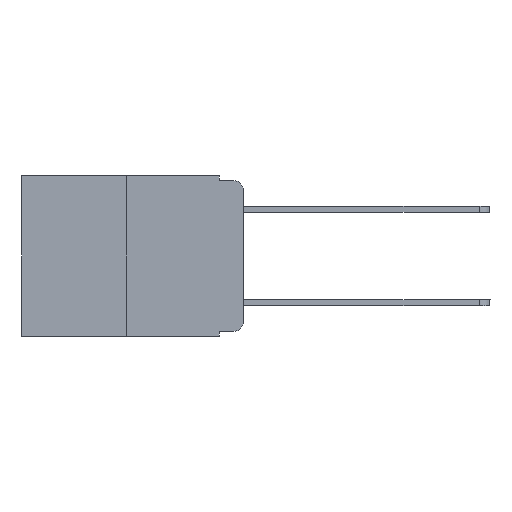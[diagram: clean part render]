
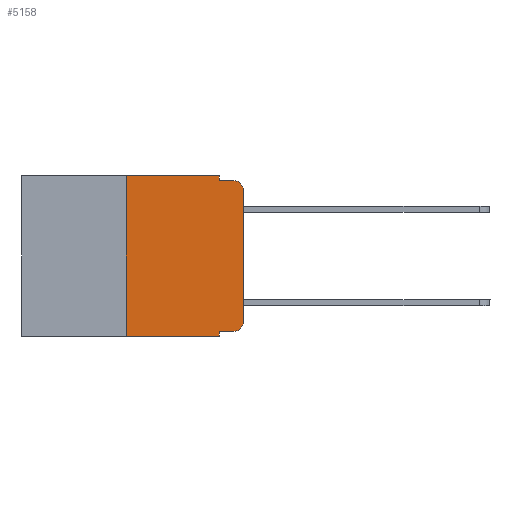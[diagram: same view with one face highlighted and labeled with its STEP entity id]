
A CAD part, left-side view. The second image highlights one B-rep face of the part: STEP entity #5158.
In plain terms, the highlighted planar face has unit normal (-1, 0, 0).
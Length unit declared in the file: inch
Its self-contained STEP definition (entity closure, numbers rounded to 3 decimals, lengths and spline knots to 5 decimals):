
#321 = EDGE_CURVE ( 'NONE', #15017, #14104, #5727, .T. ) ;
#492 = ORIENTED_EDGE ( 'NONE', *, *, #1290, .T. ) ;
#833 = ORIENTED_EDGE ( 'NONE', *, *, #7509, .F. ) ;
#1290 = EDGE_CURVE ( 'NONE', #7722, #4418, #1539, .T. ) ;
#1388 = CARTESIAN_POINT ( 'NONE',  ( 0., 0.051, -0.333 ) ) ;
#1406 = DIRECTION ( 'NONE',  ( -1., 0., 0. ) ) ;
#1539 = LINE ( 'NONE', #12666, #15130 ) ;
#1644 = VECTOR ( 'NONE', #11924, 39.37008 ) ;
#1881 = CARTESIAN_POINT ( 'NONE',  ( 0., 0., 0. ) ) ;
#1985 = FACE_OUTER_BOUND ( 'NONE', #8503, .T. ) ;
#3303 = EDGE_CURVE ( 'NONE', #15473, #14909, #5227, .T. ) ;
#3491 = CARTESIAN_POINT ( 'NONE',  ( 0., 0.02, -0.01 ) ) ;
#3507 = LINE ( 'NONE', #1388, #11747 ) ;
#3516 = AXIS2_PLACEMENT_3D ( 'NONE', #14765, #1406, #15905 ) ;
#4091 = DIRECTION ( 'NONE',  ( 0., -1., 0. ) ) ;
#4334 = CARTESIAN_POINT ( 'NONE',  ( 0., 0.051, 0. ) ) ;
#4418 = VERTEX_POINT ( 'NONE', #13692 ) ;
#4553 = DIRECTION ( 'NONE',  ( 0., -1., 0. ) ) ;
#4775 = CARTESIAN_POINT ( 'NONE',  ( 0., 0.02, -0.333 ) ) ;
#5158 = ADVANCED_FACE ( 'NONE', ( #1985 ), #9285, .F. ) ;
#5227 = LINE ( 'NONE', #11128, #7269 ) ;
#5446 = CARTESIAN_POINT ( 'NONE',  ( 0., 0.25, -0.343 ) ) ;
#5560 = ORIENTED_EDGE ( 'NONE', *, *, #16649, .F. ) ;
#5727 = CIRCLE ( 'NONE', #3516, 0.02 ) ;
#6538 = DIRECTION ( 'NONE',  ( 0., 0., 1. ) ) ;
#6646 = DIRECTION ( 'NONE',  ( 0., 0., -1. ) ) ;
#6820 = DIRECTION ( 'NONE',  ( 0., 0., -1. ) ) ;
#6831 = LINE ( 'NONE', #8954, #13431 ) ;
#7071 = CARTESIAN_POINT ( 'NONE',  ( 0., 0.25, 0. ) ) ;
#7188 = EDGE_CURVE ( 'NONE', #14104, #15911, #16356, .T. ) ;
#7213 = ORIENTED_EDGE ( 'NONE', *, *, #8533, .F. ) ;
#7269 = VECTOR ( 'NONE', #11346, 39.37008 ) ;
#7395 = LINE ( 'NONE', #10584, #1644 ) ;
#7405 = ORIENTED_EDGE ( 'NONE', *, *, #3303, .F. ) ;
#7509 = EDGE_CURVE ( 'NONE', #7722, #15473, #16743, .T. ) ;
#7722 = VERTEX_POINT ( 'NONE', #5446 ) ;
#7758 = CARTESIAN_POINT ( 'NONE',  ( 0., 0.051, -0.01 ) ) ;
#8503 = EDGE_LOOP ( 'NONE', ( #14515, #11494, #5560, #9505, #7405, #833, #492, #7213, #11826, #15370 ) ) ;
#8533 = EDGE_CURVE ( 'NONE', #13294, #4418, #6831, .T. ) ;
#8658 = VECTOR ( 'NONE', #4553, 39.37008 ) ;
#8735 = CIRCLE ( 'NONE', #11249, 0.02 ) ;
#8954 = CARTESIAN_POINT ( 'NONE',  ( 0., 0.051, 0. ) ) ;
#9285 = PLANE ( 'NONE',  #13527 ) ;
#9288 = DIRECTION ( 'NONE',  ( -1., 0., 0. ) ) ;
#9340 = EDGE_CURVE ( 'NONE', #13294, #15017, #3507, .T. ) ;
#9457 = CARTESIAN_POINT ( 'NONE',  ( 0., 0.02, -0.03 ) ) ;
#9505 = ORIENTED_EDGE ( 'NONE', *, *, #13441, .F. ) ;
#9738 = VECTOR ( 'NONE', #6538, 39.37008 ) ;
#10048 = DIRECTION ( 'NONE',  ( 0., -1., 0. ) ) ;
#10584 = CARTESIAN_POINT ( 'NONE',  ( 0., 0.051, 0. ) ) ;
#11069 = CARTESIAN_POINT ( 'NONE',  ( 0., 0., -0.313 ) ) ;
#11083 = DIRECTION ( 'NONE',  ( 0., 0., 1. ) ) ;
#11128 = CARTESIAN_POINT ( 'NONE',  ( 0., 0.473, 0. ) ) ;
#11249 = AXIS2_PLACEMENT_3D ( 'NONE', #9457, #9288, #6820 ) ;
#11288 = VERTEX_POINT ( 'NONE', #7758 ) ;
#11346 = DIRECTION ( 'NONE',  ( 0., -1., 0. ) ) ;
#11494 = ORIENTED_EDGE ( 'NONE', *, *, #14700, .T. ) ;
#11747 = VECTOR ( 'NONE', #4091, 39.37008 ) ;
#11826 = ORIENTED_EDGE ( 'NONE', *, *, #9340, .T. ) ;
#11885 = CARTESIAN_POINT ( 'NONE',  ( 0., 0.473, 0. ) ) ;
#11924 = DIRECTION ( 'NONE',  ( 0., 0., -1. ) ) ;
#11952 = CARTESIAN_POINT ( 'NONE',  ( 0., 0.25, 0. ) ) ;
#12183 = CARTESIAN_POINT ( 'NONE',  ( 0., 0., -0.03 ) ) ;
#12226 = VERTEX_POINT ( 'NONE', #3491 ) ;
#12507 = CARTESIAN_POINT ( 'NONE',  ( 0., 0.051, -0.01 ) ) ;
#12666 = CARTESIAN_POINT ( 'NONE',  ( 0., 0.473, -0.343 ) ) ;
#12933 = DIRECTION ( 'NONE',  ( 0., 0., -1. ) ) ;
#13020 = CARTESIAN_POINT ( 'NONE',  ( 0., 0.051, -0.333 ) ) ;
#13211 = DIRECTION ( 'NONE',  ( 1., 0., 0. ) ) ;
#13294 = VERTEX_POINT ( 'NONE', #13020 ) ;
#13431 = VECTOR ( 'NONE', #12933, 39.37008 ) ;
#13441 = EDGE_CURVE ( 'NONE', #14909, #11288, #7395, .T. ) ;
#13527 = AXIS2_PLACEMENT_3D ( 'NONE', #11885, #13211, #6646 ) ;
#13692 = CARTESIAN_POINT ( 'NONE',  ( 0., 0.051, -0.343 ) ) ;
#13843 = LINE ( 'NONE', #12507, #8658 ) ;
#14104 = VERTEX_POINT ( 'NONE', #11069 ) ;
#14515 = ORIENTED_EDGE ( 'NONE', *, *, #7188, .T. ) ;
#14700 = EDGE_CURVE ( 'NONE', #15911, #12226, #8735, .T. ) ;
#14765 = CARTESIAN_POINT ( 'NONE',  ( 0., 0.02, -0.313 ) ) ;
#14909 = VERTEX_POINT ( 'NONE', #4334 ) ;
#15017 = VERTEX_POINT ( 'NONE', #4775 ) ;
#15130 = VECTOR ( 'NONE', #10048, 39.37008 ) ;
#15370 = ORIENTED_EDGE ( 'NONE', *, *, #321, .T. ) ;
#15473 = VERTEX_POINT ( 'NONE', #7071 ) ;
#15905 = DIRECTION ( 'NONE',  ( 0., 0., -1. ) ) ;
#15911 = VERTEX_POINT ( 'NONE', #12183 ) ;
#16141 = VECTOR ( 'NONE', #11083, 39.37008 ) ;
#16356 = LINE ( 'NONE', #1881, #16141 ) ;
#16649 = EDGE_CURVE ( 'NONE', #11288, #12226, #13843, .T. ) ;
#16743 = LINE ( 'NONE', #11952, #9738 ) ;
